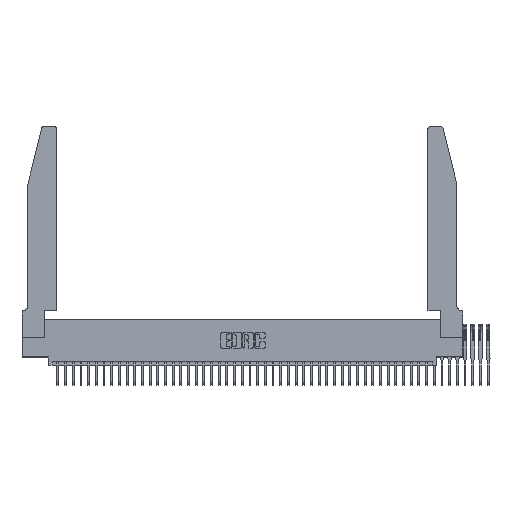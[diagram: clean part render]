
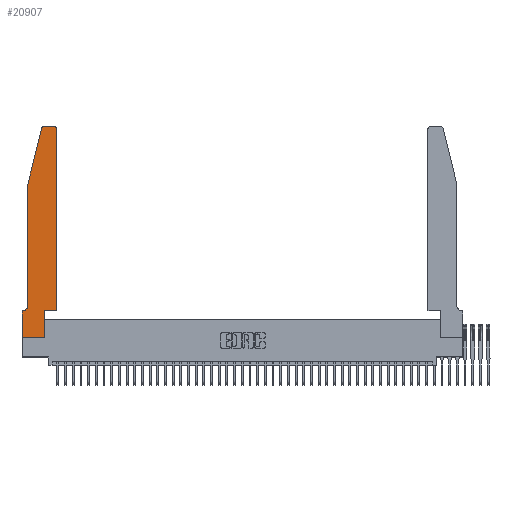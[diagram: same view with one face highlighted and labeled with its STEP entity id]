
A CAD part, top view. The second image highlights one B-rep face of the part: STEP entity #20907.
In plain terms, the highlighted planar face has unit normal (0, 0, 1).
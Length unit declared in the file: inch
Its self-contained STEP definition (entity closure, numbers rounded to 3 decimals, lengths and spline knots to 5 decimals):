
#581 = CIRCLE ( 'NONE', #39874, 0.07 ) ;
#1354 = DIRECTION ( 'NONE',  ( 1., 0., 0. ) ) ;
#2143 = VERTEX_POINT ( 'NONE', #9516 ) ;
#2835 = EDGE_CURVE ( 'NONE', #40945, #17379, #21491, .T. ) ;
#3159 = VERTEX_POINT ( 'NONE', #30781 ) ;
#4155 = CARTESIAN_POINT ( 'NONE',  ( 0.4205, 2.72, 0.37 ) ) ;
#4724 = VECTOR ( 'NONE', #40221, 39.37008 ) ;
#4978 = DIRECTION ( 'NONE',  ( 0., 0., 1. ) ) ;
#5671 = LINE ( 'NONE', #8892, #30038 ) ;
#5792 = EDGE_CURVE ( 'NONE', #17379, #32952, #15775, .T. ) ;
#6022 = VERTEX_POINT ( 'NONE', #27848 ) ;
#6141 = DIRECTION ( 'NONE',  ( 1., 0., 0. ) ) ;
#6328 = DIRECTION ( 'NONE',  ( 0., -1., 0. ) ) ;
#6330 = ORIENTED_EDGE ( 'NONE', *, *, #7996, .T. ) ;
#6347 = VERTEX_POINT ( 'NONE', #35919 ) ;
#6747 = VERTEX_POINT ( 'NONE', #31659 ) ;
#7382 = DIRECTION ( 'NONE',  ( 1., 0., 0. ) ) ;
#7490 = VECTOR ( 'NONE', #29137, 39.37008 ) ;
#7996 = EDGE_CURVE ( 'NONE', #6747, #40945, #38851, .T. ) ;
#8488 = LINE ( 'NONE', #25968, #7490 ) ;
#8862 = ORIENTED_EDGE ( 'NONE', *, *, #17271, .T. ) ;
#8892 = CARTESIAN_POINT ( 'NONE',  ( 0.0755, 2., 0.37 ) ) ;
#9496 = ORIENTED_EDGE ( 'NONE', *, *, #29554, .T. ) ;
#9516 = CARTESIAN_POINT ( 'NONE',  ( 0.0755, 0.42, 0.37 ) ) ;
#9580 = ORIENTED_EDGE ( 'NONE', *, *, #28775, .T. ) ;
#10362 = CARTESIAN_POINT ( 'NONE',  ( 0.2865, 0., 0.37 ) ) ;
#10639 = EDGE_LOOP ( 'NONE', ( #9496, #29367, #15540, #9580, #28457, #13358, #11847, #6330, #16823, #22814, #8862, #27782 ) ) ;
#11777 = VECTOR ( 'NONE', #35966, 39.37008 ) ;
#11847 = ORIENTED_EDGE ( 'NONE', *, *, #39008, .T. ) ;
#13099 = VECTOR ( 'NONE', #38251, 39.37008 ) ;
#13358 = ORIENTED_EDGE ( 'NONE', *, *, #39229, .T. ) ;
#13549 = LINE ( 'NONE', #25418, #30343 ) ;
#13649 = VECTOR ( 'NONE', #6141, 39.37008 ) ;
#13721 = CARTESIAN_POINT ( 'NONE',  ( 0.4505, 0.35, 0.37 ) ) ;
#14148 = PLANE ( 'NONE',  #30568 ) ;
#14272 = LINE ( 'NONE', #37085, #4724 ) ;
#15540 = ORIENTED_EDGE ( 'NONE', *, *, #28231, .T. ) ;
#15775 = LINE ( 'NONE', #20232, #11777 ) ;
#16823 = ORIENTED_EDGE ( 'NONE', *, *, #2835, .T. ) ;
#17108 = CARTESIAN_POINT ( 'NONE',  ( 0.0055, 0.42, 0.37 ) ) ;
#17271 = EDGE_CURVE ( 'NONE', #32952, #3159, #14272, .T. ) ;
#17276 = VECTOR ( 'NONE', #39904, 39.37008 ) ;
#17379 = VERTEX_POINT ( 'NONE', #28140 ) ;
#17877 = VERTEX_POINT ( 'NONE', #29097 ) ;
#18778 = CARTESIAN_POINT ( 'NONE',  ( 0.284, 2.75, 0.37 ) ) ;
#19766 = LINE ( 'NONE', #28242, #35588 ) ;
#20232 = CARTESIAN_POINT ( 'NONE',  ( 0.4505, 0.35, 0.37 ) ) ;
#20306 = DIRECTION ( 'NONE',  ( -1., 0., 0. ) ) ;
#20510 = DIRECTION ( 'NONE',  ( 0., 0., 1. ) ) ;
#20907 = ADVANCED_FACE ( 'NONE', ( #25443 ), #14148, .T. ) ;
#21491 = LINE ( 'NONE', #22244, #13099 ) ;
#21724 = AXIS2_PLACEMENT_3D ( 'NONE', #24096, #4978, #27282 ) ;
#21774 = VERTEX_POINT ( 'NONE', #28350 ) ;
#21782 = VERTEX_POINT ( 'NONE', #18778 ) ;
#22244 = CARTESIAN_POINT ( 'NONE',  ( 0.2865, 0.35, 0.37 ) ) ;
#22315 = VERTEX_POINT ( 'NONE', #28185 ) ;
#22814 = ORIENTED_EDGE ( 'NONE', *, *, #5792, .T. ) ;
#23047 = CIRCLE ( 'NONE', #21724, 0.03 ) ;
#23585 = CARTESIAN_POINT ( 'NONE',  ( 0., 0.35, 0.37 ) ) ;
#24096 = CARTESIAN_POINT ( 'NONE',  ( 0.284, 2.72, 0.37 ) ) ;
#24103 = CARTESIAN_POINT ( 'NONE',  ( 0., 0., 0.37 ) ) ;
#25273 = EDGE_CURVE ( 'NONE', #3159, #6347, #25386, .T. ) ;
#25386 = CIRCLE ( 'NONE', #35526, 0.03 ) ;
#25418 = CARTESIAN_POINT ( 'NONE',  ( 0.0755, 2., 0.37 ) ) ;
#25443 = FACE_OUTER_BOUND ( 'NONE', #10639, .T. ) ;
#25752 = LINE ( 'NONE', #24103, #17276 ) ;
#25968 = CARTESIAN_POINT ( 'NONE',  ( 0.2605, 2.75, 0.37 ) ) ;
#26466 = DIRECTION ( 'NONE',  ( 0., 0., 1. ) ) ;
#27282 = DIRECTION ( 'NONE',  ( 1., 0., 0. ) ) ;
#27782 = ORIENTED_EDGE ( 'NONE', *, *, #25273, .T. ) ;
#27848 = CARTESIAN_POINT ( 'NONE',  ( 0.0755, 2., 0.37 ) ) ;
#27948 = DIRECTION ( 'NONE',  ( -0.239, -0.971, 0. ) ) ;
#28140 = CARTESIAN_POINT ( 'NONE',  ( 0.2865, 0.35, 0.37 ) ) ;
#28185 = CARTESIAN_POINT ( 'NONE',  ( 0.0055, 0.35, 0.37 ) ) ;
#28231 = EDGE_CURVE ( 'NONE', #17877, #6022, #5671, .T. ) ;
#28242 = CARTESIAN_POINT ( 'NONE',  ( 0.0755, 0.35, 0.37 ) ) ;
#28350 = CARTESIAN_POINT ( 'NONE',  ( 0., 0.35, 0.37 ) ) ;
#28399 = CARTESIAN_POINT ( 'NONE',  ( 0., 0., 0.37 ) ) ;
#28457 = ORIENTED_EDGE ( 'NONE', *, *, #33687, .T. ) ;
#28775 = EDGE_CURVE ( 'NONE', #6022, #2143, #13549, .T. ) ;
#29097 = CARTESIAN_POINT ( 'NONE',  ( 0.25487, 2.72718, 0.37 ) ) ;
#29137 = DIRECTION ( 'NONE',  ( -1., 0., 0. ) ) ;
#29367 = ORIENTED_EDGE ( 'NONE', *, *, #35814, .T. ) ;
#29554 = EDGE_CURVE ( 'NONE', #6347, #21782, #8488, .T. ) ;
#30038 = VECTOR ( 'NONE', #27948, 39.37008 ) ;
#30343 = VECTOR ( 'NONE', #6328, 39.37008 ) ;
#30568 = AXIS2_PLACEMENT_3D ( 'NONE', #23585, #20510, #1354 ) ;
#30781 = CARTESIAN_POINT ( 'NONE',  ( 0.4505, 2.72, 0.37 ) ) ;
#31403 = DIRECTION ( 'NONE',  ( -1., 0., 0. ) ) ;
#31659 = CARTESIAN_POINT ( 'NONE',  ( 0., 0., 0.37 ) ) ;
#32952 = VERTEX_POINT ( 'NONE', #13721 ) ;
#33687 = EDGE_CURVE ( 'NONE', #2143, #22315, #581, .T. ) ;
#35526 = AXIS2_PLACEMENT_3D ( 'NONE', #4155, #26466, #7382 ) ;
#35588 = VECTOR ( 'NONE', #31403, 39.37008 ) ;
#35814 = EDGE_CURVE ( 'NONE', #21782, #17877, #23047, .T. ) ;
#35919 = CARTESIAN_POINT ( 'NONE',  ( 0.4205, 2.75, 0.37 ) ) ;
#35966 = DIRECTION ( 'NONE',  ( 1., 0., 0. ) ) ;
#37085 = CARTESIAN_POINT ( 'NONE',  ( 0.4505, 0.35, 0.37 ) ) ;
#38251 = DIRECTION ( 'NONE',  ( 0., 1., 0. ) ) ;
#38851 = LINE ( 'NONE', #28399, #13649 ) ;
#39008 = EDGE_CURVE ( 'NONE', #21774, #6747, #25752, .T. ) ;
#39195 = DIRECTION ( 'NONE',  ( 0., 0., -1. ) ) ;
#39229 = EDGE_CURVE ( 'NONE', #22315, #21774, #19766, .T. ) ;
#39874 = AXIS2_PLACEMENT_3D ( 'NONE', #17108, #39195, #20306 ) ;
#39904 = DIRECTION ( 'NONE',  ( 0., -1., 0. ) ) ;
#40221 = DIRECTION ( 'NONE',  ( 0., 1., 0. ) ) ;
#40945 = VERTEX_POINT ( 'NONE', #10362 ) ;
